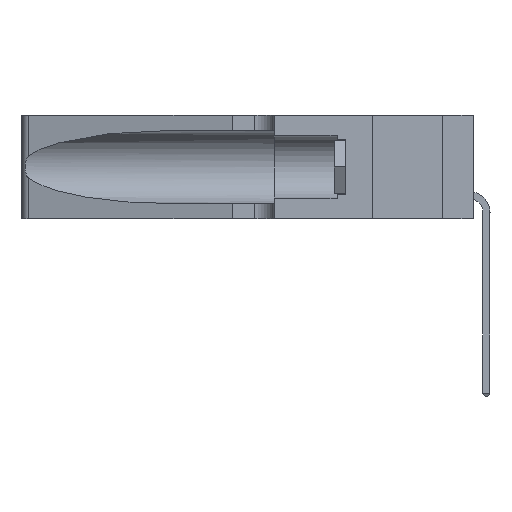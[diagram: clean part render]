
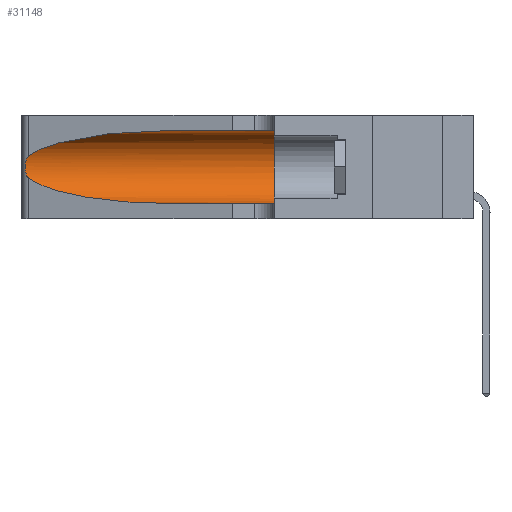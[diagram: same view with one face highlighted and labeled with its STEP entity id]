
A CAD part, left-side view. The second image highlights one B-rep face of the part: STEP entity #31148.
In plain terms, the highlighted cylindrical face has radius 3.308 mm (diameter 6.617 mm), a partial arc.
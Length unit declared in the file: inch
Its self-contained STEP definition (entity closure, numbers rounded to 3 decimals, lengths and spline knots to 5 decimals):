
#604 = DIRECTION ( 'NONE',  ( 0., 0., 1. ) ) ;
#923 = VERTEX_POINT ( 'NONE', #41977 ) ;
#1307 = CARTESIAN_POINT ( 'NONE',  ( 0.1305, 1.61858, 0.05475 ) ) ;
#1693 = CARTESIAN_POINT ( 'NONE',  ( 0.25639, 1.23184, 0.21858 ) ) ;
#2118 = LINE ( 'NONE', #1307, #18854 ) ;
#2332 = CARTESIAN_POINT ( 'NONE',  ( 0.1305, 0.72297, 0.31525 ) ) ;
#2420 = AXIS2_PLACEMENT_3D ( 'NONE', #23122, #3698, #6981 ) ;
#2877 = VERTEX_POINT ( 'NONE', #6441 ) ;
#3698 = DIRECTION ( 'NONE',  ( 0., -1., 0. ) ) ;
#3711 = CIRCLE ( 'NONE', #41086, 0.13025 ) ;
#3716 = ORIENTED_EDGE ( 'NONE', *, *, #8519, .T. ) ;
#5240 = CARTESIAN_POINT ( 'NONE',  ( 0.25487, 1.22718, 0.14631 ) ) ;
#5694 = CARTESIAN_POINT ( 'NONE',  ( 0.26018, 1.23835, 0.19895 ) ) ;
#5769 = CARTESIAN_POINT ( 'NONE',  ( 0.25487, 1.22718, 0.14631 ) ) ;
#5829 = CARTESIAN_POINT ( 'NONE',  ( 0.26075, 1.23896, 0.178 ) ) ;
#5914 = CARTESIAN_POINT ( 'NONE',  ( 0.1305, 0.35, 0.05475 ) ) ;
#6032 = CARTESIAN_POINT ( 'NONE',  ( 0.1305, 0.72297, 0.05475 ) ) ;
#6301 = VECTOR ( 'NONE', #40399, 39.37008 ) ;
#6429 = EDGE_CURVE ( 'NONE', #7799, #2877, #36105, .T. ) ;
#6441 = CARTESIAN_POINT ( 'NONE',  ( 0.1305, 0.35, 0.31525 ) ) ;
#6981 = DIRECTION ( 'NONE',  ( 0., 0., -1. ) ) ;
#7718 = EDGE_CURVE ( 'NONE', #12511, #21310, #2118, .T. ) ;
#7799 = VERTEX_POINT ( 'NONE', #15756 ) ;
#8358 = FACE_OUTER_BOUND ( 'NONE', #22655, .T. ) ;
#8519 = EDGE_CURVE ( 'NONE', #7799, #923, #10599, .T. ) ;
#8861 = ORIENTED_EDGE ( 'NONE', *, *, #23432, .T. ) ;
#9107 = CARTESIAN_POINT ( 'NONE',  ( 0.25856, 1.23593, 0.16098 ) ) ;
#9818 = EDGE_CURVE ( 'NONE', #923, #36267, #37130, .T. ) ;
#10237 = ORIENTED_EDGE ( 'NONE', *, *, #18172, .F. ) ;
#10343 = CYLINDRICAL_SURFACE ( 'NONE', #2420, 0.13025 ) ;
#10599 =( BOUNDED_CURVE ( )  B_SPLINE_CURVE ( 3, ( #2332, #34920, #15925, #22581 ),
 .UNSPECIFIED., .F., .T. ) 
 B_SPLINE_CURVE_WITH_KNOTS ( ( 4, 4 ),
 ( 1.5708, 2.84003 ),
 .UNSPECIFIED. ) 
 CURVE ( )  GEOMETRIC_REPRESENTATION_ITEM ( )  RATIONAL_B_SPLINE_CURVE ( ( 1., 0.87, 0.87, 1. ) ) 
 REPRESENTATION_ITEM ( '' )  );
#12511 = VERTEX_POINT ( 'NONE', #6032 ) ;
#14740 = ORIENTED_EDGE ( 'NONE', *, *, #7718, .T. ) ;
#15014 = CARTESIAN_POINT ( 'NONE',  ( 0.25787, 1.23484, 0.2124 ) ) ;
#15756 = CARTESIAN_POINT ( 'NONE',  ( 0.1305, 0.72297, 0.31525 ) ) ;
#15925 = CARTESIAN_POINT ( 'NONE',  ( 0.2373, 1.15595, 0.28018 ) ) ;
#16155 = CARTESIAN_POINT ( 'NONE',  ( 0.25555, 1.22993, 0.14849 ) ) ;
#18172 = EDGE_CURVE ( 'NONE', #2877, #21310, #3711, .T. ) ;
#18695 =( BOUNDED_CURVE ( )  B_SPLINE_CURVE ( 3, ( #5769, #26320, #25206, #31706 ),
 .UNSPECIFIED., .F., .F. ) 
 B_SPLINE_CURVE_WITH_KNOTS ( ( 4, 4 ),
 ( 3.44316, 4.71239 ),
 .UNSPECIFIED. ) 
 CURVE ( )  GEOMETRIC_REPRESENTATION_ITEM ( )  RATIONAL_B_SPLINE_CURVE ( ( 1., 0.87, 0.87, 1. ) ) 
 REPRESENTATION_ITEM ( '' )  );
#18854 = VECTOR ( 'NONE', #37050, 39.37008 ) ;
#21310 = VERTEX_POINT ( 'NONE', #5914 ) ;
#22273 = CARTESIAN_POINT ( 'NONE',  ( 0.26017, 1.23833, 0.17102 ) ) ;
#22581 = CARTESIAN_POINT ( 'NONE',  ( 0.25487, 1.22718, 0.22369 ) ) ;
#22655 = EDGE_LOOP ( 'NONE', ( #3716, #36495, #8861, #14740, #10237, #36883 ) ) ;
#23122 = CARTESIAN_POINT ( 'NONE',  ( 0.1305, 1.61858, 0.185 ) ) ;
#23432 = EDGE_CURVE ( 'NONE', #36267, #12511, #18695, .T. ) ;
#25206 = CARTESIAN_POINT ( 'NONE',  ( 0.18966, 0.96281, 0.05475 ) ) ;
#26320 = CARTESIAN_POINT ( 'NONE',  ( 0.2373, 1.15595, 0.08982 ) ) ;
#27103 = CARTESIAN_POINT ( 'NONE',  ( 0.1305, 1.61858, 0.31525 ) ) ;
#28686 = CARTESIAN_POINT ( 'NONE',  ( 0.25789, 1.23486, 0.15765 ) ) ;
#31148 = ADVANCED_FACE ( 'NONE', ( #8358 ), #10343, .F. ) ;
#31480 = CARTESIAN_POINT ( 'NONE',  ( 0.26075, 1.23896, 0.19203 ) ) ;
#31706 = CARTESIAN_POINT ( 'NONE',  ( 0.1305, 0.72297, 0.05475 ) ) ;
#34450 = CARTESIAN_POINT ( 'NONE',  ( 0.25487, 1.22718, 0.22369 ) ) ;
#34920 = CARTESIAN_POINT ( 'NONE',  ( 0.18966, 0.96281, 0.31525 ) ) ;
#35692 = CARTESIAN_POINT ( 'NONE',  ( 0.25639, 1.23186, 0.15144 ) ) ;
#35821 = CARTESIAN_POINT ( 'NONE',  ( 0.25487, 1.22718, 0.14631 ) ) ;
#36105 = LINE ( 'NONE', #27103, #6301 ) ;
#36267 = VERTEX_POINT ( 'NONE', #5240 ) ;
#36495 = ORIENTED_EDGE ( 'NONE', *, *, #9818, .T. ) ;
#36803 = DIRECTION ( 'NONE',  ( 0., 1., 0. ) ) ;
#36883 = ORIENTED_EDGE ( 'NONE', *, *, #6429, .F. ) ;
#37050 = DIRECTION ( 'NONE',  ( 0., -1., 0. ) ) ;
#37130 = B_SPLINE_CURVE_WITH_KNOTS ( 'NONE', 3,
 ( #34450, #40534, #1693, #15014, #37447, #5694, #31480, #5829, #22273, #9107, #28686, #35692, #16155, #35821 ),
 .UNSPECIFIED., .F., .F.,
 ( 4, 2, 2, 2, 2, 2, 4 ),
 ( 0., 0.00027, 0.00053, 0.00107, 0.0016, 0.00187, 0.00214 ),
 .UNSPECIFIED. ) ;
#37447 = CARTESIAN_POINT ( 'NONE',  ( 0.25854, 1.2359, 0.20912 ) ) ;
#39486 = CARTESIAN_POINT ( 'NONE',  ( 0.1305, 0.35, 0.185 ) ) ;
#40399 = DIRECTION ( 'NONE',  ( 0., -1., 0. ) ) ;
#40534 = CARTESIAN_POINT ( 'NONE',  ( 0.25555, 1.22994, 0.2215 ) ) ;
#41086 = AXIS2_PLACEMENT_3D ( 'NONE', #39486, #36803, #604 ) ;
#41977 = CARTESIAN_POINT ( 'NONE',  ( 0.25487, 1.22718, 0.22369 ) ) ;
